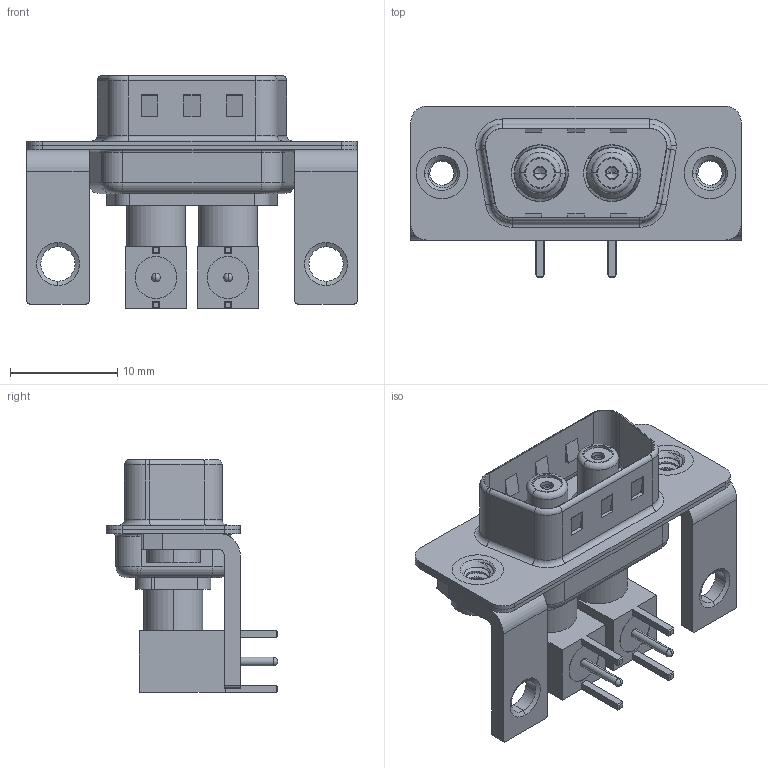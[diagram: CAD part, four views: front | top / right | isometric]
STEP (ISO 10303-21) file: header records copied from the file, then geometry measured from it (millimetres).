
FILE_DESCRIPTION (( 'STEP AP203' ), '1' );
FILE_NAME ('629-2W2-640-5TC.STEP', '2022-05-04T22:49:56', ( '' ), ( '' ), 'SwSTEP 2.0', 'SolidWorks 2020', '' );
FILE_SCHEMA (( 'CONFIG_CONTROL_DESIGN' ));
Length unit declared in the file: millimetre
Products named in the file (15): 629-2W2-640-5TC; 629Combo Stabilizer Bracket; Locking Collar; Insulator RA Pin; 629Combo Threaded Rivet_2; Socket_RA; Insulator Socket; 629Combo Housing_2W2; 629Combo Shell Rear_09 Contacts; Co-Ax Jack Assy_RA; Insulator Socket 2; RA Back Shell; Co-Ax Jack_RA PC Tail; 629Combo Shell Front_09 Contacts
Assembly tree (23 placements, depth 3):
  629-2W2-640-5TC
    629Combo Housing_2W2
    629Combo Shell Rear_09 Contacts
    629Combo Shell Front_09 Contacts
    629Combo Threaded Rivet_2  x2
    629Combo Stabilizer Bracket  x2
    Co-Ax Jack Assy_RA
      Co-Ax Jack_RA PC Tail
      Insulator Socket
      Insulator Socket 2
      Locking Collar
      Socket_RA
      RA Back Shell
      Insulator RA Pin
    Co-Ax Jack Assy_RA
      Co-Ax Jack_RA PC Tail
      Insulator Socket
      Insulator Socket 2
      Locking Collar
      Socket_RA
      RA Back Shell
      Insulator RA Pin
Bounding box: 30.8 x 16 x 21.71 mm (x, y, z)
Volume: 2194.5 mm3; surface area: 6106.6 mm2
Topology: 21 solids, 21 shells, 656 faces, 1575 edges, 984 vertices
Faces by surface type: cylinder 287, plane 241, torus 62, cone 54, bspline 8, sphere 4
Entity records: 16710 total; most frequent: CARTESIAN_POINT 3978, DIRECTION 2440, ORIENTED_EDGE 2170, EDGE_CURVE 1085, AXIS2_PLACEMENT_3D 944, VERTEX_POINT 683, VECTOR 552, LINE 552
